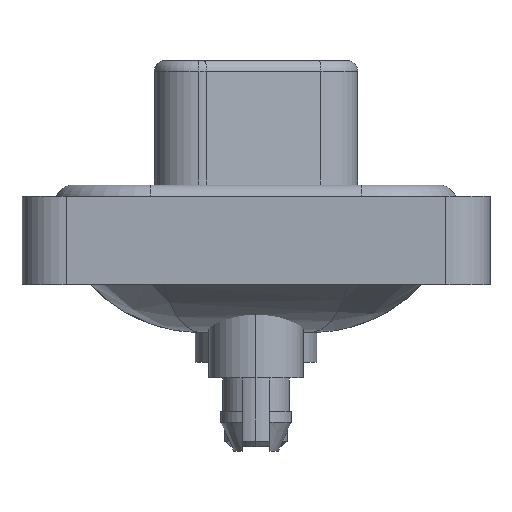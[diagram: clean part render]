
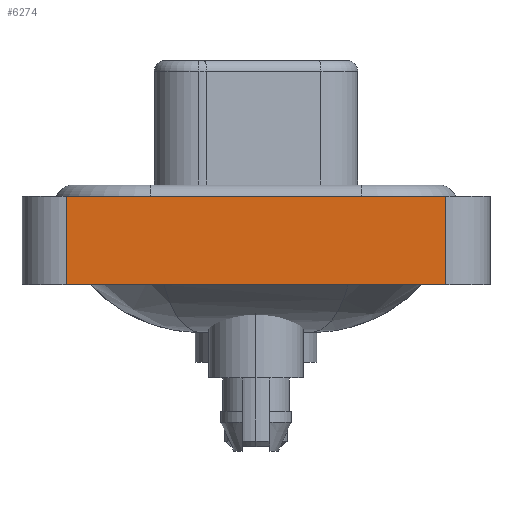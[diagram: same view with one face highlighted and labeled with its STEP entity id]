
A CAD part, left-side view. The second image highlights one B-rep face of the part: STEP entity #6274.
In plain terms, the highlighted planar face has unit normal (-1, 0, 0).
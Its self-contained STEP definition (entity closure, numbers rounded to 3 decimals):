
#322 = VERTEX_POINT ( 'NONE', #9919 ) ;
#573 = DIRECTION ( 'NONE',  ( 0., 0., 1. ) ) ;
#927 = ORIENTED_EDGE ( 'NONE', *, *, #17461, .T. ) ;
#1448 = LINE ( 'NONE', #8972, #20051 ) ;
#3886 = CARTESIAN_POINT ( 'NONE',  ( -7.25, -8.55, 0.4 ) ) ;
#4784 = VECTOR ( 'NONE', #20033, 1000. ) ;
#5549 = VERTEX_POINT ( 'NONE', #8537 ) ;
#5695 = VECTOR ( 'NONE', #573, 1000. ) ;
#6274 = ADVANCED_FACE ( 'NONE', ( #15777 ), #17097, .T. ) ;
#6440 = CARTESIAN_POINT ( 'NONE',  ( -7.25, -8.55, -3.6 ) ) ;
#6532 = DIRECTION ( 'NONE',  ( -1., 0., 0. ) ) ;
#6797 = ORIENTED_EDGE ( 'NONE', *, *, #18661, .T. ) ;
#6863 = CARTESIAN_POINT ( 'NONE',  ( -7.25, -8.55, -3.6 ) ) ;
#6915 = VECTOR ( 'NONE', #9732, 1000. ) ;
#7257 = VERTEX_POINT ( 'NONE', #6863 ) ;
#7757 = DIRECTION ( 'NONE',  ( 0., 0., 1. ) ) ;
#7851 = CARTESIAN_POINT ( 'NONE',  ( -7.25, -8.55, -3.6 ) ) ;
#8537 = CARTESIAN_POINT ( 'NONE',  ( -7.25, 8.55, -3.6 ) ) ;
#8972 = CARTESIAN_POINT ( 'NONE',  ( -7.25, -8.55, -3.6 ) ) ;
#9649 = ORIENTED_EDGE ( 'NONE', *, *, #10505, .F. ) ;
#9732 = DIRECTION ( 'NONE',  ( 0., -1., 0. ) ) ;
#9919 = CARTESIAN_POINT ( 'NONE',  ( -7.25, 8.55, 0.4 ) ) ;
#10505 = EDGE_CURVE ( 'NONE', #322, #18575, #11552, .T. ) ;
#11552 = LINE ( 'NONE', #16211, #6915 ) ;
#14043 = LINE ( 'NONE', #7851, #4784 ) ;
#15054 = ORIENTED_EDGE ( 'NONE', *, *, #15939, .F. ) ;
#15777 = FACE_OUTER_BOUND ( 'NONE', #18100, .T. ) ;
#15939 = EDGE_CURVE ( 'NONE', #5549, #322, #17528, .T. ) ;
#16211 = CARTESIAN_POINT ( 'NONE',  ( -7.25, -8.55, 0.4 ) ) ;
#16777 = DIRECTION ( 'NONE',  ( 0., 0., 1. ) ) ;
#17097 = PLANE ( 'NONE',  #17827 ) ;
#17461 = EDGE_CURVE ( 'NONE', #7257, #18575, #1448, .T. ) ;
#17528 = LINE ( 'NONE', #19074, #5695 ) ;
#17827 = AXIS2_PLACEMENT_3D ( 'NONE', #6440, #6532, #7757 ) ;
#18100 = EDGE_LOOP ( 'NONE', ( #927, #9649, #15054, #6797 ) ) ;
#18575 = VERTEX_POINT ( 'NONE', #3886 ) ;
#18661 = EDGE_CURVE ( 'NONE', #5549, #7257, #14043, .T. ) ;
#19074 = CARTESIAN_POINT ( 'NONE',  ( -7.25, 8.55, -3.6 ) ) ;
#20033 = DIRECTION ( 'NONE',  ( 0., -1., 0. ) ) ;
#20051 = VECTOR ( 'NONE', #16777, 1000. ) ;
